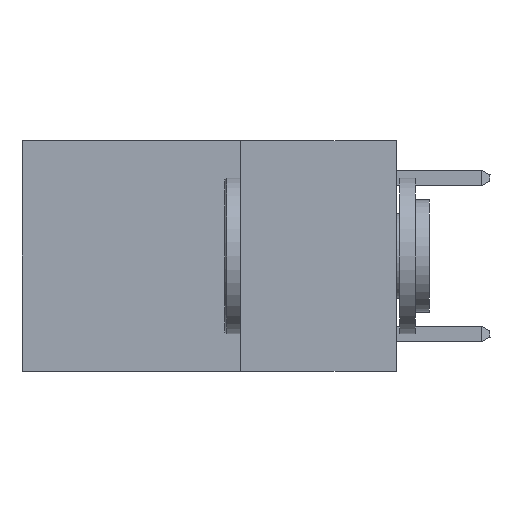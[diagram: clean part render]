
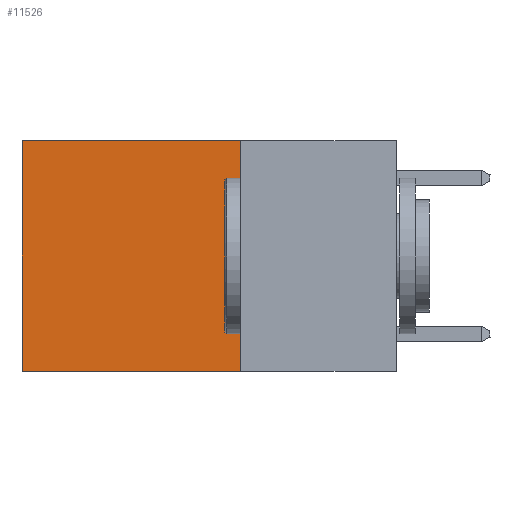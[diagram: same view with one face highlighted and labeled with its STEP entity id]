
A CAD part, left-side view. The second image highlights one B-rep face of the part: STEP entity #11526.
In plain terms, the highlighted planar face has unit normal (-1, 0, 0).
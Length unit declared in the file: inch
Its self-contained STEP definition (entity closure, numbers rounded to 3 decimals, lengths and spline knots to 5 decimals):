
#273 = VECTOR ( 'NONE', #11206, 39.37008 ) ;
#958 = CARTESIAN_POINT ( 'NONE',  ( 0.2625, 0.25, 0. ) ) ;
#1100 = VERTEX_POINT ( 'NONE', #3454 ) ;
#1132 = VECTOR ( 'NONE', #6176, 39.37008 ) ;
#1434 = LINE ( 'NONE', #8926, #1132 ) ;
#2395 = AXIS2_PLACEMENT_3D ( 'NONE', #3826, #9416, #2934 ) ;
#2570 = EDGE_CURVE ( 'NONE', #10444, #1100, #12041, .T. ) ;
#2934 = DIRECTION ( 'NONE',  ( 0., 0., -1. ) ) ;
#3454 = CARTESIAN_POINT ( 'NONE',  ( 0.2625, 0.6, -0.37 ) ) ;
#3826 = CARTESIAN_POINT ( 'NONE',  ( 0.2625, 0.25, 0. ) ) ;
#4208 = LINE ( 'NONE', #11857, #5376 ) ;
#4399 = CARTESIAN_POINT ( 'NONE',  ( 0.2625, 0.25, -0.37 ) ) ;
#4459 = EDGE_CURVE ( 'NONE', #10931, #10707, #1434, .T. ) ;
#4562 = CARTESIAN_POINT ( 'NONE',  ( 0.2625, 0.25, 0. ) ) ;
#5376 = VECTOR ( 'NONE', #10917, 39.37008 ) ;
#5388 = ORIENTED_EDGE ( 'NONE', *, *, #2570, .F. ) ;
#5924 = CARTESIAN_POINT ( 'NONE',  ( 0.2625, 0.6, 0. ) ) ;
#6176 = DIRECTION ( 'NONE',  ( 0., 1., 0. ) ) ;
#6273 = LINE ( 'NONE', #4562, #6636 ) ;
#6391 = DIRECTION ( 'NONE',  ( 0., 0., -1. ) ) ;
#6503 = EDGE_LOOP ( 'NONE', ( #8970, #5388, #7111, #9446 ) ) ;
#6636 = VECTOR ( 'NONE', #6391, 39.37008 ) ;
#7111 = ORIENTED_EDGE ( 'NONE', *, *, #11808, .F. ) ;
#7785 = PLANE ( 'NONE',  #2395 ) ;
#8388 = CARTESIAN_POINT ( 'NONE',  ( 0.2625, 0.25, -0.37 ) ) ;
#8926 = CARTESIAN_POINT ( 'NONE',  ( 0.2625, 0.25, 0. ) ) ;
#8970 = ORIENTED_EDGE ( 'NONE', *, *, #9502, .T. ) ;
#9416 = DIRECTION ( 'NONE',  ( 1., 0., 0. ) ) ;
#9446 = ORIENTED_EDGE ( 'NONE', *, *, #4459, .T. ) ;
#9502 = EDGE_CURVE ( 'NONE', #10707, #1100, #4208, .T. ) ;
#10444 = VERTEX_POINT ( 'NONE', #4399 ) ;
#10707 = VERTEX_POINT ( 'NONE', #5924 ) ;
#10917 = DIRECTION ( 'NONE',  ( 0., 0., -1. ) ) ;
#10931 = VERTEX_POINT ( 'NONE', #958 ) ;
#11206 = DIRECTION ( 'NONE',  ( 0., 1., 0. ) ) ;
#11526 = ADVANCED_FACE ( 'NONE', ( #12382 ), #7785, .F. ) ;
#11808 = EDGE_CURVE ( 'NONE', #10931, #10444, #6273, .T. ) ;
#11857 = CARTESIAN_POINT ( 'NONE',  ( 0.2625, 0.6, 0. ) ) ;
#12041 = LINE ( 'NONE', #8388, #273 ) ;
#12382 = FACE_OUTER_BOUND ( 'NONE', #6503, .T. ) ;
